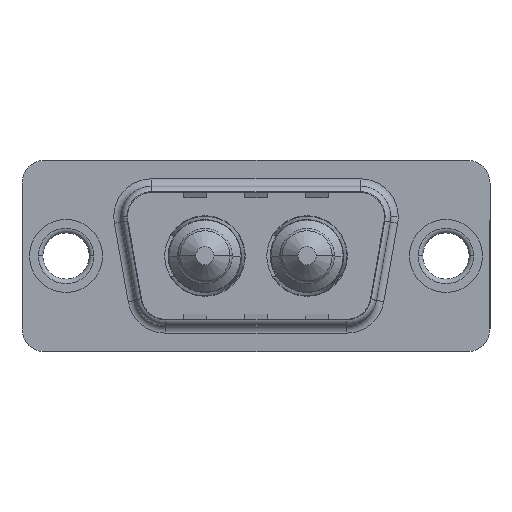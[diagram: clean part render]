
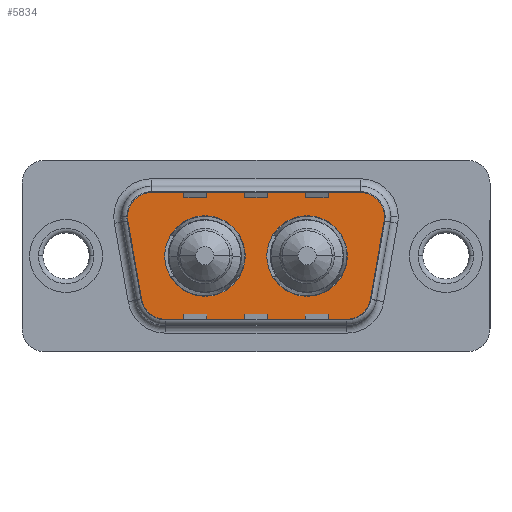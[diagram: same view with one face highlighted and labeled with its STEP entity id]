
A CAD part, top view. The second image highlights one B-rep face of the part: STEP entity #5834.
In plain terms, the highlighted planar face has unit normal (0, 0, 1).
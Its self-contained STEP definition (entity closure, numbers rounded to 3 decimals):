
#64 = AXIS2_PLACEMENT_3D ( 'NONE', #5937, #3820, #4976 ) ;
#169 = LINE ( 'NONE', #3029, #3987 ) ;
#233 = DIRECTION ( 'NONE',  ( -1., 0., 0. ) ) ;
#550 = ORIENTED_EDGE ( 'NONE', *, *, #6584, .T. ) ;
#557 = CARTESIAN_POINT ( 'NONE',  ( 6.49, 0., 0. ) ) ;
#635 = DIRECTION ( 'NONE',  ( 1., 0., 0. ) ) ;
#657 = CARTESIAN_POINT ( 'NONE',  ( 21.534, 2.553, 0. ) ) ;
#868 = CARTESIAN_POINT ( 'NONE',  ( 15.86, 0., 0. ) ) ;
#911 = VERTEX_POINT ( 'NONE', #3230 ) ;
#1243 = CARTESIAN_POINT ( 'NONE',  ( 19.564, 2.9, 0. ) ) ;
#1259 = CARTESIAN_POINT ( 'NONE',  ( 18.541, -2.9, 0. ) ) ;
#1520 = EDGE_CURVE ( 'NONE', #4649, #5450, #7824, .T. ) ;
#1570 = DIRECTION ( 'NONE',  ( 0.174, -0.985, 0. ) ) ;
#1769 = DIRECTION ( 'NONE',  ( 1., 0., 0. ) ) ;
#1792 = AXIS2_PLACEMENT_3D ( 'NONE', #2943, #7611, #7807 ) ;
#1985 = AXIS2_PLACEMENT_3D ( 'NONE', #1243, #2441, #233 ) ;
#1998 = VERTEX_POINT ( 'NONE', #2636 ) ;
#2169 = AXIS2_PLACEMENT_3D ( 'NONE', #4867, #6260, #6102 ) ;
#2370 = ORIENTED_EDGE ( 'NONE', *, *, #3698, .T. ) ;
#2441 = DIRECTION ( 'NONE',  ( 0., 0., 1. ) ) ;
#2621 = EDGE_CURVE ( 'NONE', #9255, #6641, #5584, .T. ) ;
#2636 = CARTESIAN_POINT ( 'NONE',  ( 6.459, -4.9, 0. ) ) ;
#2702 = AXIS2_PLACEMENT_3D ( 'NONE', #4346, #4688, #4252 ) ;
#2710 = AXIS2_PLACEMENT_3D ( 'NONE', #4403, #6977, #6704 ) ;
#2773 = ORIENTED_EDGE ( 'NONE', *, *, #2621, .T. ) ;
#2943 = CARTESIAN_POINT ( 'NONE',  ( 9.14, 0., 0. ) ) ;
#2953 = EDGE_CURVE ( 'NONE', #5450, #7398, #169, .T. ) ;
#3029 = CARTESIAN_POINT ( 'NONE',  ( 5.436, 4.9, 0. ) ) ;
#3042 = AXIS2_PLACEMENT_3D ( 'NONE', #6120, #8441, #635 ) ;
#3118 = VECTOR ( 'NONE', #5468, 1000. ) ;
#3131 = VECTOR ( 'NONE', #8117, 1000. ) ;
#3230 = CARTESIAN_POINT ( 'NONE',  ( 13.21, 0., 0. ) ) ;
#3355 = LINE ( 'NONE', #6418, #3131 ) ;
#3449 = ORIENTED_EDGE ( 'NONE', *, *, #6339, .T. ) ;
#3462 = CIRCLE ( 'NONE', #2169, 2.65 ) ;
#3469 = CARTESIAN_POINT ( 'NONE',  ( 18.51, 0., 0. ) ) ;
#3476 = CARTESIAN_POINT ( 'NONE',  ( 21.564, 2.9, 0. ) ) ;
#3547 = ORIENTED_EDGE ( 'NONE', *, *, #4145, .T. ) ;
#3560 = PLANE ( 'NONE',  #5116 ) ;
#3568 = EDGE_LOOP ( 'NONE', ( #9400, #7856 ) ) ;
#3698 = EDGE_CURVE ( 'NONE', #8605, #4649, #8768, .T. ) ;
#3820 = DIRECTION ( 'NONE',  ( 0., 0., 1. ) ) ;
#3824 = FACE_OUTER_BOUND ( 'NONE', #7024, .T. ) ;
#3987 = VECTOR ( 'NONE', #6208, 1000. ) ;
#4145 = EDGE_CURVE ( 'NONE', #7398, #9255, #8754, .T. ) ;
#4252 = DIRECTION ( 'NONE',  ( -1., 0., 0. ) ) ;
#4346 = CARTESIAN_POINT ( 'NONE',  ( 19.564, 2.9, 0. ) ) ;
#4362 = ORIENTED_EDGE ( 'NONE', *, *, #8101, .T. ) ;
#4403 = CARTESIAN_POINT ( 'NONE',  ( 15.86, 0., 0. ) ) ;
#4454 = ORIENTED_EDGE ( 'NONE', *, *, #6556, .F. ) ;
#4649 = VERTEX_POINT ( 'NONE', #3476 ) ;
#4688 = DIRECTION ( 'NONE',  ( 0., 0., 1. ) ) ;
#4748 = CARTESIAN_POINT ( 'NONE',  ( 20.511, -3.247, 0. ) ) ;
#4867 = CARTESIAN_POINT ( 'NONE',  ( 9.14, 0., 0. ) ) ;
#4976 = DIRECTION ( 'NONE',  ( 1., 0., 0. ) ) ;
#5020 = VERTEX_POINT ( 'NONE', #557 ) ;
#5071 = DIRECTION ( 'NONE',  ( -1., 0., 0. ) ) ;
#5116 = AXIS2_PLACEMENT_3D ( 'NONE', #1259, #5907, #9098 ) ;
#5233 = CARTESIAN_POINT ( 'NONE',  ( 3.466, 2.553, 0. ) ) ;
#5302 = VERTEX_POINT ( 'NONE', #4748 ) ;
#5328 = DIRECTION ( 'NONE',  ( 0., 0., 1. ) ) ;
#5450 = VERTEX_POINT ( 'NONE', #5719 ) ;
#5460 = CIRCLE ( 'NONE', #2710, 2.65 ) ;
#5466 = DIRECTION ( 'NONE',  ( 0., 0., 1. ) ) ;
#5468 = DIRECTION ( 'NONE',  ( 0.174, 0.985, 0. ) ) ;
#5473 = EDGE_CURVE ( 'NONE', #6641, #1998, #6976, .T. ) ;
#5584 = LINE ( 'NONE', #7552, #9544 ) ;
#5719 = CARTESIAN_POINT ( 'NONE',  ( 19.564, 4.9, 0. ) ) ;
#5745 = VERTEX_POINT ( 'NONE', #3469 ) ;
#5748 = CARTESIAN_POINT ( 'NONE',  ( 5.436, 4.9, 0. ) ) ;
#5834 = ADVANCED_FACE ( 'NONE', ( #7912, #7449, #3824 ), #3560, .T. ) ;
#5835 = EDGE_CURVE ( 'NONE', #5745, #911, #5460, .T. ) ;
#5857 = VERTEX_POINT ( 'NONE', #6815 ) ;
#5907 = DIRECTION ( 'NONE',  ( 0., 0., 1. ) ) ;
#5937 = CARTESIAN_POINT ( 'NONE',  ( 5.436, 2.9, 0. ) ) ;
#6098 = VERTEX_POINT ( 'NONE', #9046 ) ;
#6102 = DIRECTION ( 'NONE',  ( 1., 0., 0. ) ) ;
#6120 = CARTESIAN_POINT ( 'NONE',  ( 18.541, -2.9, 0. ) ) ;
#6208 = DIRECTION ( 'NONE',  ( -1., 0., 0. ) ) ;
#6260 = DIRECTION ( 'NONE',  ( 0., 0., 1. ) ) ;
#6264 = EDGE_CURVE ( 'NONE', #5020, #5857, #8153, .T. ) ;
#6338 = ORIENTED_EDGE ( 'NONE', *, *, #2953, .T. ) ;
#6339 = EDGE_CURVE ( 'NONE', #5302, #8605, #8931, .T. ) ;
#6418 = CARTESIAN_POINT ( 'NONE',  ( 6.459, -4.9, 0. ) ) ;
#6556 = EDGE_CURVE ( 'NONE', #911, #5745, #7685, .T. ) ;
#6584 = EDGE_CURVE ( 'NONE', #1998, #6098, #3355, .T. ) ;
#6641 = VERTEX_POINT ( 'NONE', #7179 ) ;
#6704 = DIRECTION ( 'NONE',  ( 1., 0., 0. ) ) ;
#6815 = CARTESIAN_POINT ( 'NONE',  ( 11.79, 0., 0. ) ) ;
#6823 = CARTESIAN_POINT ( 'NONE',  ( 6.459, -2.9, 0. ) ) ;
#6882 = CARTESIAN_POINT ( 'NONE',  ( 21.534, 2.553, 0. ) ) ;
#6976 = CIRCLE ( 'NONE', #7320, 2. ) ;
#6977 = DIRECTION ( 'NONE',  ( 0., 0., 1. ) ) ;
#7024 = EDGE_LOOP ( 'NONE', ( #4362, #3449, #2370, #7584, #6338, #3547, #2773, #8954, #550 ) ) ;
#7179 = CARTESIAN_POINT ( 'NONE',  ( 4.489, -3.247, 0. ) ) ;
#7320 = AXIS2_PLACEMENT_3D ( 'NONE', #6823, #5466, #5071 ) ;
#7398 = VERTEX_POINT ( 'NONE', #5748 ) ;
#7449 = FACE_BOUND ( 'NONE', #3568, .T. ) ;
#7552 = CARTESIAN_POINT ( 'NONE',  ( 3.466, 2.553, 0. ) ) ;
#7556 = AXIS2_PLACEMENT_3D ( 'NONE', #868, #5328, #1769 ) ;
#7584 = ORIENTED_EDGE ( 'NONE', *, *, #1520, .T. ) ;
#7611 = DIRECTION ( 'NONE',  ( 0., 0., 1. ) ) ;
#7685 = CIRCLE ( 'NONE', #7556, 2.65 ) ;
#7807 = DIRECTION ( 'NONE',  ( 1., 0., 0. ) ) ;
#7824 = CIRCLE ( 'NONE', #2702, 2. ) ;
#7850 = EDGE_CURVE ( 'NONE', #5857, #5020, #3462, .T. ) ;
#7856 = ORIENTED_EDGE ( 'NONE', *, *, #6264, .F. ) ;
#7912 = FACE_BOUND ( 'NONE', #8129, .T. ) ;
#8101 = EDGE_CURVE ( 'NONE', #6098, #5302, #9622, .T. ) ;
#8117 = DIRECTION ( 'NONE',  ( 1., 0., 0. ) ) ;
#8129 = EDGE_LOOP ( 'NONE', ( #9111, #4454 ) ) ;
#8153 = CIRCLE ( 'NONE', #1792, 2.65 ) ;
#8441 = DIRECTION ( 'NONE',  ( 0., 0., 1. ) ) ;
#8605 = VERTEX_POINT ( 'NONE', #657 ) ;
#8754 = CIRCLE ( 'NONE', #64, 2. ) ;
#8768 = CIRCLE ( 'NONE', #1985, 2. ) ;
#8931 = LINE ( 'NONE', #6882, #3118 ) ;
#8954 = ORIENTED_EDGE ( 'NONE', *, *, #5473, .T. ) ;
#9046 = CARTESIAN_POINT ( 'NONE',  ( 18.541, -4.9, 0. ) ) ;
#9098 = DIRECTION ( 'NONE',  ( 1., 0., 0. ) ) ;
#9111 = ORIENTED_EDGE ( 'NONE', *, *, #5835, .F. ) ;
#9255 = VERTEX_POINT ( 'NONE', #5233 ) ;
#9400 = ORIENTED_EDGE ( 'NONE', *, *, #7850, .F. ) ;
#9544 = VECTOR ( 'NONE', #1570, 1000. ) ;
#9622 = CIRCLE ( 'NONE', #3042, 2. ) ;
